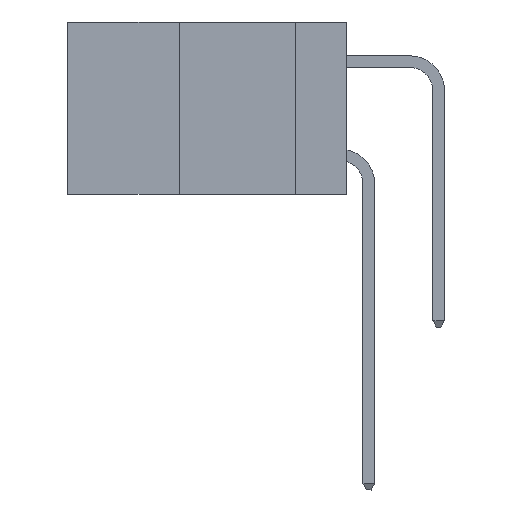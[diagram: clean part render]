
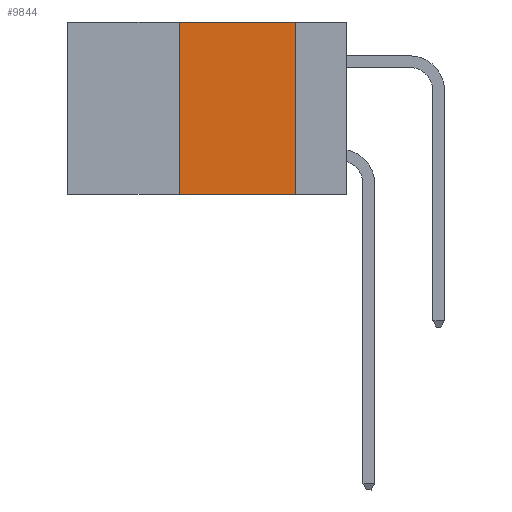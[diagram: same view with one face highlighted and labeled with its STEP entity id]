
A CAD part, left-side view. The second image highlights one B-rep face of the part: STEP entity #9844.
In plain terms, the highlighted planar face has unit normal (-1, 0, 0).
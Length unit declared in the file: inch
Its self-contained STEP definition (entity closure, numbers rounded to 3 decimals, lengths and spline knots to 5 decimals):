
#15 = EDGE_CURVE ( 'NONE', #4068, #12881, #10804, .T. ) ;
#306 = FACE_OUTER_BOUND ( 'NONE', #765, .T. ) ;
#646 = LINE ( 'NONE', #4881, #1483 ) ;
#765 = EDGE_LOOP ( 'NONE', ( #7755, #1269, #10405, #6848 ) ) ;
#1269 = ORIENTED_EDGE ( 'NONE', *, *, #11661, .F. ) ;
#1483 = VECTOR ( 'NONE', #13339, 39.37008 ) ;
#1495 = VERTEX_POINT ( 'NONE', #3379 ) ;
#1877 = DIRECTION ( 'NONE',  ( 0., 0., -1. ) ) ;
#2142 = EDGE_CURVE ( 'NONE', #1495, #13378, #4171, .T. ) ;
#2470 = DIRECTION ( 'NONE',  ( 1., 0., 0. ) ) ;
#3030 = LINE ( 'NONE', #7129, #8245 ) ;
#3379 = CARTESIAN_POINT ( 'NONE',  ( 0., 0.11, 0. ) ) ;
#3575 = PLANE ( 'NONE',  #5689 ) ;
#3717 = CARTESIAN_POINT ( 'NONE',  ( 0., 0.6, 0. ) ) ;
#4062 = DIRECTION ( 'NONE',  ( 0., -1., 0. ) ) ;
#4068 = VERTEX_POINT ( 'NONE', #12688 ) ;
#4171 = LINE ( 'NONE', #7370, #4344 ) ;
#4344 = VECTOR ( 'NONE', #1877, 39.37008 ) ;
#4881 = CARTESIAN_POINT ( 'NONE',  ( 0., 0.6, 0. ) ) ;
#5525 = DIRECTION ( 'NONE',  ( 0., 0., 1. ) ) ;
#5689 = AXIS2_PLACEMENT_3D ( 'NONE', #3717, #2470, #12044 ) ;
#6848 = ORIENTED_EDGE ( 'NONE', *, *, #10738, .T. ) ;
#7129 = CARTESIAN_POINT ( 'NONE',  ( 0., 0.6, -0.37 ) ) ;
#7370 = CARTESIAN_POINT ( 'NONE',  ( 0., 0.11, 0. ) ) ;
#7755 = ORIENTED_EDGE ( 'NONE', *, *, #2142, .F. ) ;
#8245 = VECTOR ( 'NONE', #4062, 39.37008 ) ;
#9844 = ADVANCED_FACE ( 'NONE', ( #306 ), #3575, .F. ) ;
#10405 = ORIENTED_EDGE ( 'NONE', *, *, #15, .F. ) ;
#10738 = EDGE_CURVE ( 'NONE', #4068, #13378, #3030, .T. ) ;
#10804 = LINE ( 'NONE', #10874, #11608 ) ;
#10874 = CARTESIAN_POINT ( 'NONE',  ( 0., 0.36, 0. ) ) ;
#11133 = CARTESIAN_POINT ( 'NONE',  ( 0., 0.36, 0. ) ) ;
#11608 = VECTOR ( 'NONE', #5525, 39.37008 ) ;
#11661 = EDGE_CURVE ( 'NONE', #12881, #1495, #646, .T. ) ;
#12044 = DIRECTION ( 'NONE',  ( 0., 0., -1. ) ) ;
#12346 = CARTESIAN_POINT ( 'NONE',  ( 0., 0.11, -0.37 ) ) ;
#12688 = CARTESIAN_POINT ( 'NONE',  ( 0., 0.36, -0.37 ) ) ;
#12881 = VERTEX_POINT ( 'NONE', #11133 ) ;
#13339 = DIRECTION ( 'NONE',  ( 0., -1., 0. ) ) ;
#13378 = VERTEX_POINT ( 'NONE', #12346 ) ;
